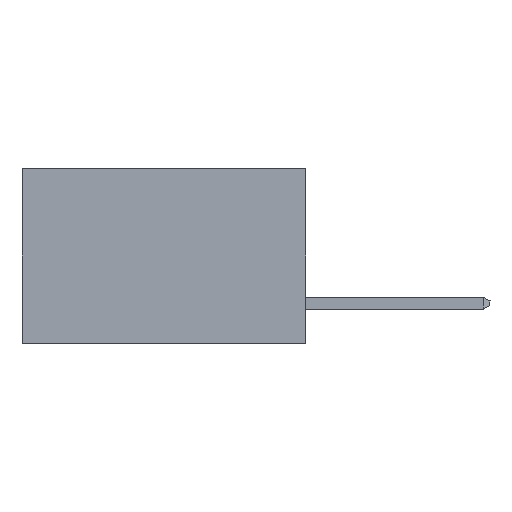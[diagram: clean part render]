
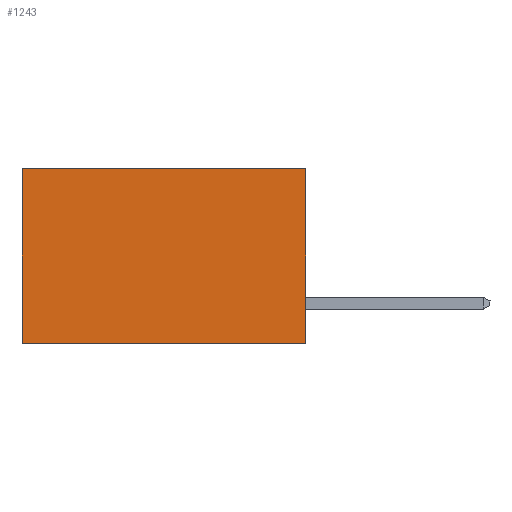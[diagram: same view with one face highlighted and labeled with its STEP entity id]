
A CAD part, left-side view. The second image highlights one B-rep face of the part: STEP entity #1243.
In plain terms, the highlighted planar face has unit normal (-1, 0, 0).
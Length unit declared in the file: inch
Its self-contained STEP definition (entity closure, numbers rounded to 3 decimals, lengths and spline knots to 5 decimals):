
#103 = LINE ( 'NONE', #18057, #11439 ) ;
#476 = LINE ( 'NONE', #5046, #8751 ) ;
#1243 = ADVANCED_FACE ( 'NONE', ( #4128 ), #13743, .F. ) ;
#2341 = ORIENTED_EDGE ( 'NONE', *, *, #10385, .T. ) ;
#3100 = LINE ( 'NONE', #19759, #14756 ) ;
#4128 = FACE_OUTER_BOUND ( 'NONE', #9431, .T. ) ;
#4981 = DIRECTION ( 'NONE',  ( 0., 0., -1. ) ) ;
#5046 = CARTESIAN_POINT ( 'NONE',  ( 0.298, 0., -0.37 ) ) ;
#5646 = CARTESIAN_POINT ( 'NONE',  ( 0.298, 0., 0. ) ) ;
#6784 = EDGE_CURVE ( 'NONE', #9244, #23367, #476, .T. ) ;
#7155 = ORIENTED_EDGE ( 'NONE', *, *, #16585, .T. ) ;
#8751 = VECTOR ( 'NONE', #18029, 39.37008 ) ;
#9054 = DIRECTION ( 'NONE',  ( 1., 0., 0. ) ) ;
#9237 = CARTESIAN_POINT ( 'NONE',  ( 0.298, 0., 0. ) ) ;
#9244 = VERTEX_POINT ( 'NONE', #17363 ) ;
#9250 = ORIENTED_EDGE ( 'NONE', *, *, #6784, .F. ) ;
#9431 = EDGE_LOOP ( 'NONE', ( #2341, #9250, #26298, #7155 ) ) ;
#10385 = EDGE_CURVE ( 'NONE', #12245, #23367, #103, .T. ) ;
#10735 = LINE ( 'NONE', #5646, #26261 ) ;
#11439 = VECTOR ( 'NONE', #4981, 39.37008 ) ;
#12245 = VERTEX_POINT ( 'NONE', #16461 ) ;
#12386 = AXIS2_PLACEMENT_3D ( 'NONE', #9237, #9054, #15789 ) ;
#12750 = DIRECTION ( 'NONE',  ( 0., 1., 0. ) ) ;
#13743 = PLANE ( 'NONE',  #12386 ) ;
#14643 = CARTESIAN_POINT ( 'NONE',  ( 0.298, 0., 0. ) ) ;
#14756 = VECTOR ( 'NONE', #12750, 39.37008 ) ;
#15789 = DIRECTION ( 'NONE',  ( 0., 0., -1. ) ) ;
#16409 = CARTESIAN_POINT ( 'NONE',  ( 0.298, 0.6, -0.37 ) ) ;
#16461 = CARTESIAN_POINT ( 'NONE',  ( 0.298, 0.6, 0. ) ) ;
#16585 = EDGE_CURVE ( 'NONE', #28023, #12245, #3100, .T. ) ;
#16814 = DIRECTION ( 'NONE',  ( 0., 0., -1. ) ) ;
#17363 = CARTESIAN_POINT ( 'NONE',  ( 0.298, 0., -0.37 ) ) ;
#18029 = DIRECTION ( 'NONE',  ( 0., 1., 0. ) ) ;
#18057 = CARTESIAN_POINT ( 'NONE',  ( 0.298, 0.6, 0. ) ) ;
#19759 = CARTESIAN_POINT ( 'NONE',  ( 0.298, 0., 0. ) ) ;
#23367 = VERTEX_POINT ( 'NONE', #16409 ) ;
#26261 = VECTOR ( 'NONE', #16814, 39.37008 ) ;
#26298 = ORIENTED_EDGE ( 'NONE', *, *, #27990, .F. ) ;
#27990 = EDGE_CURVE ( 'NONE', #28023, #9244, #10735, .T. ) ;
#28023 = VERTEX_POINT ( 'NONE', #14643 ) ;
